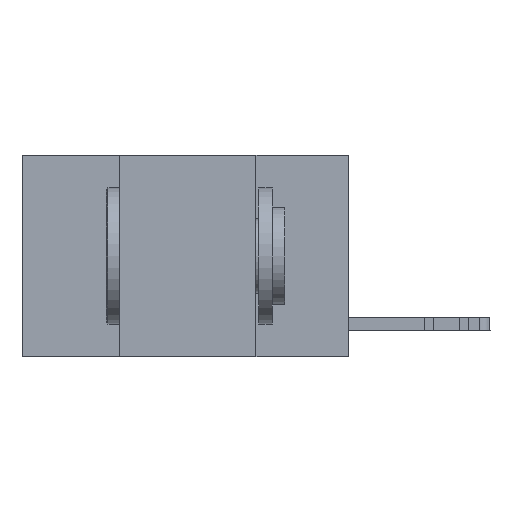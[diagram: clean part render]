
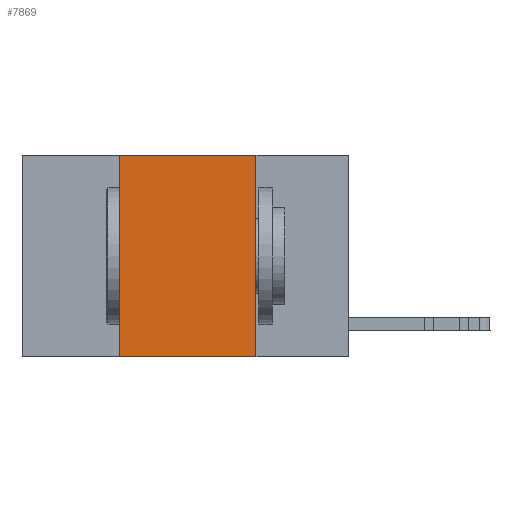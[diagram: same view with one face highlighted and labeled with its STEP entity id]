
A CAD part, left-side view. The second image highlights one B-rep face of the part: STEP entity #7869.
In plain terms, the highlighted planar face has unit normal (-1, 0, 0).
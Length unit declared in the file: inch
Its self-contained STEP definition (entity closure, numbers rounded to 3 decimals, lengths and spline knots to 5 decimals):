
#1544 = CARTESIAN_POINT ( 'NONE',  ( 0., 0.42, -0.37 ) ) ;
#2625 = AXIS2_PLACEMENT_3D ( 'NONE', #15448, #17504, #10701 ) ;
#2801 = ORIENTED_EDGE ( 'NONE', *, *, #28906, .T. ) ;
#2812 = ORIENTED_EDGE ( 'NONE', *, *, #14795, .F. ) ;
#2846 = CARTESIAN_POINT ( 'NONE',  ( 0., 0.6, 0. ) ) ;
#5114 = ORIENTED_EDGE ( 'NONE', *, *, #25891, .F. ) ;
#5197 = CARTESIAN_POINT ( 'NONE',  ( 0., 0.42, 0. ) ) ;
#5914 = DIRECTION ( 'NONE',  ( 0., 0., -1. ) ) ;
#6794 = ORIENTED_EDGE ( 'NONE', *, *, #17758, .F. ) ;
#6906 = VECTOR ( 'NONE', #22779, 39.37008 ) ;
#7407 = LINE ( 'NONE', #5197, #26198 ) ;
#7869 = ADVANCED_FACE ( 'NONE', ( #8617 ), #19846, .F. ) ;
#8564 = CARTESIAN_POINT ( 'NONE',  ( 0., 0.6, -0.37 ) ) ;
#8617 = FACE_OUTER_BOUND ( 'NONE', #27741, .T. ) ;
#8849 = LINE ( 'NONE', #8564, #20614 ) ;
#9126 = VECTOR ( 'NONE', #5914, 39.37008 ) ;
#10701 = DIRECTION ( 'NONE',  ( 0., 0., -1. ) ) ;
#10838 = CARTESIAN_POINT ( 'NONE',  ( 0., 0.17, 0. ) ) ;
#11079 = VERTEX_POINT ( 'NONE', #23040 ) ;
#14795 = EDGE_CURVE ( 'NONE', #23185, #27608, #17147, .T. ) ;
#15448 = CARTESIAN_POINT ( 'NONE',  ( 0., 0.6, 0. ) ) ;
#17147 = LINE ( 'NONE', #26144, #9126 ) ;
#17504 = DIRECTION ( 'NONE',  ( 1., 0., 0. ) ) ;
#17740 = DIRECTION ( 'NONE',  ( 0., -1., 0. ) ) ;
#17758 = EDGE_CURVE ( 'NONE', #27201, #11079, #7407, .T. ) ;
#19846 = PLANE ( 'NONE',  #2625 ) ;
#20614 = VECTOR ( 'NONE', #17740, 39.37008 ) ;
#22779 = DIRECTION ( 'NONE',  ( 0., -1., 0. ) ) ;
#23040 = CARTESIAN_POINT ( 'NONE',  ( 0., 0.42, 0. ) ) ;
#23078 = DIRECTION ( 'NONE',  ( 0., 0., 1. ) ) ;
#23080 = LINE ( 'NONE', #2846, #6906 ) ;
#23185 = VERTEX_POINT ( 'NONE', #10838 ) ;
#25891 = EDGE_CURVE ( 'NONE', #11079, #23185, #23080, .T. ) ;
#26144 = CARTESIAN_POINT ( 'NONE',  ( 0., 0.17, 0. ) ) ;
#26198 = VECTOR ( 'NONE', #23078, 39.37008 ) ;
#27201 = VERTEX_POINT ( 'NONE', #1544 ) ;
#27608 = VERTEX_POINT ( 'NONE', #29070 ) ;
#27741 = EDGE_LOOP ( 'NONE', ( #2812, #5114, #6794, #2801 ) ) ;
#28906 = EDGE_CURVE ( 'NONE', #27201, #27608, #8849, .T. ) ;
#29070 = CARTESIAN_POINT ( 'NONE',  ( 0., 0.17, -0.37 ) ) ;
